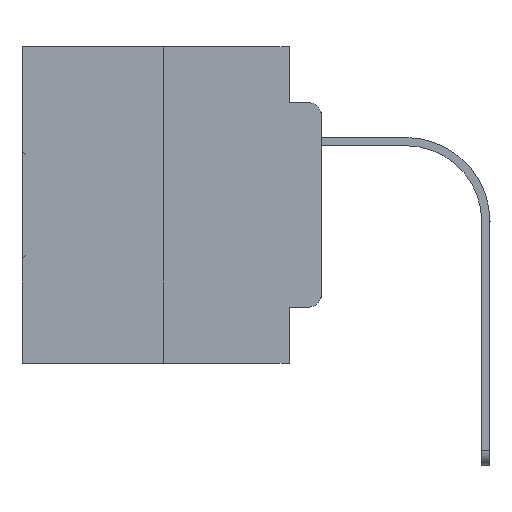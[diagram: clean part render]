
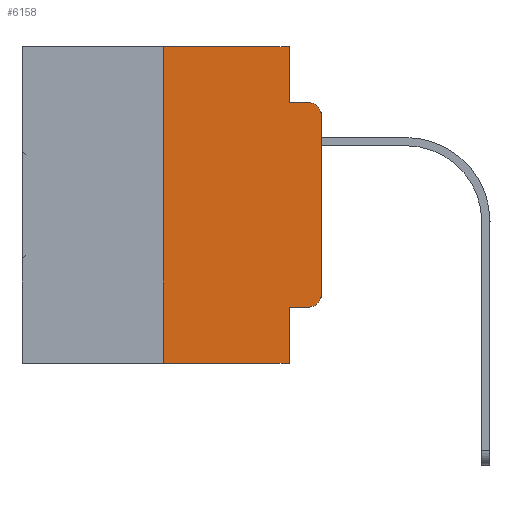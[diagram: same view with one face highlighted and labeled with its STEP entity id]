
A CAD part, left-side view. The second image highlights one B-rep face of the part: STEP entity #6158.
In plain terms, the highlighted planar face has unit normal (-1, 0, 0).
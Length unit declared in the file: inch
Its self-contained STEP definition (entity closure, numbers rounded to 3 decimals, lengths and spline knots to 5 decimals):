
#133 = EDGE_CURVE ( 'NONE', #17402, #2380, #21622, .T. ) ;
#395 = VECTOR ( 'NONE', #9404, 39.37008 ) ;
#664 = CARTESIAN_POINT ( 'NONE',  ( 0., 0.25, 0. ) ) ;
#854 = LINE ( 'NONE', #12624, #10473 ) ;
#1053 = EDGE_CURVE ( 'NONE', #10923, #3500, #10325, .T. ) ;
#1316 = DIRECTION ( 'NONE',  ( 0., 0., 1. ) ) ;
#1574 = VECTOR ( 'NONE', #30043, 39.37008 ) ;
#2047 = ORIENTED_EDGE ( 'NONE', *, *, #26265, .T. ) ;
#2172 = CARTESIAN_POINT ( 'NONE',  ( 0., 0., -0.1085 ) ) ;
#2380 = VERTEX_POINT ( 'NONE', #4368 ) ;
#2775 = EDGE_CURVE ( 'NONE', #23478, #12491, #9440, .T. ) ;
#3223 = EDGE_CURVE ( 'NONE', #12491, #11195, #23045, .T. ) ;
#3500 = VERTEX_POINT ( 'NONE', #2172 ) ;
#3657 = EDGE_CURVE ( 'NONE', #11195, #26979, #28485, .T. ) ;
#4109 = LINE ( 'NONE', #8973, #10966 ) ;
#4368 = CARTESIAN_POINT ( 'NONE',  ( 0., 0.051, -0.5 ) ) ;
#6158 = ADVANCED_FACE ( 'NONE', ( #27324 ), #6329, .F. ) ;
#6208 = ORIENTED_EDGE ( 'NONE', *, *, #1053, .T. ) ;
#6329 = PLANE ( 'NONE',  #11194 ) ;
#6498 = DIRECTION ( 'NONE',  ( -1., 0., 0. ) ) ;
#7035 = ORIENTED_EDGE ( 'NONE', *, *, #133, .F. ) ;
#7985 = LINE ( 'NONE', #17350, #1574 ) ;
#8927 = CARTESIAN_POINT ( 'NONE',  ( 0., 0.473, 0. ) ) ;
#8973 = CARTESIAN_POINT ( 'NONE',  ( 0., 0.25, 0. ) ) ;
#9230 = DIRECTION ( 'NONE',  ( -1., 0., 0. ) ) ;
#9243 = CARTESIAN_POINT ( 'NONE',  ( 0., 0.051, 0. ) ) ;
#9404 = DIRECTION ( 'NONE',  ( 0., 0., -1. ) ) ;
#9440 = LINE ( 'NONE', #26138, #26828 ) ;
#9497 = CIRCLE ( 'NONE', #17349, 0.02 ) ;
#9725 = CARTESIAN_POINT ( 'NONE',  ( 0., 0.051, 0. ) ) ;
#10325 = LINE ( 'NONE', #24876, #26907 ) ;
#10331 = CIRCLE ( 'NONE', #17681, 0.02 ) ;
#10473 = VECTOR ( 'NONE', #21947, 39.37008 ) ;
#10923 = VERTEX_POINT ( 'NONE', #30077 ) ;
#10943 = EDGE_CURVE ( 'NONE', #3500, #26979, #10331, .T. ) ;
#10966 = VECTOR ( 'NONE', #13126, 39.37008 ) ;
#11194 = AXIS2_PLACEMENT_3D ( 'NONE', #8927, #15665, #25036 ) ;
#11195 = VERTEX_POINT ( 'NONE', #17194 ) ;
#11224 = EDGE_CURVE ( 'NONE', #28524, #2380, #7985, .T. ) ;
#11507 = ORIENTED_EDGE ( 'NONE', *, *, #3223, .F. ) ;
#11794 = ORIENTED_EDGE ( 'NONE', *, *, #11224, .T. ) ;
#12491 = VERTEX_POINT ( 'NONE', #9725 ) ;
#12624 = CARTESIAN_POINT ( 'NONE',  ( 0., 0.051, -0.4115 ) ) ;
#13034 = CARTESIAN_POINT ( 'NONE',  ( 0., 0.051, -0.4115 ) ) ;
#13126 = DIRECTION ( 'NONE',  ( 0., 0., 1. ) ) ;
#13244 = CARTESIAN_POINT ( 'NONE',  ( 0., 0.02, -0.3915 ) ) ;
#13622 = CARTESIAN_POINT ( 'NONE',  ( 0., 0.25, -0.5 ) ) ;
#15005 = ORIENTED_EDGE ( 'NONE', *, *, #10943, .T. ) ;
#15176 = CARTESIAN_POINT ( 'NONE',  ( 0., 0.051, 0. ) ) ;
#15540 = EDGE_CURVE ( 'NONE', #28363, #10923, #9497, .T. ) ;
#15665 = DIRECTION ( 'NONE',  ( 1., 0., 0. ) ) ;
#16259 = VECTOR ( 'NONE', #26185, 39.37008 ) ;
#17194 = CARTESIAN_POINT ( 'NONE',  ( 0., 0.051, -0.0885 ) ) ;
#17349 = AXIS2_PLACEMENT_3D ( 'NONE', #13244, #6498, #29330 ) ;
#17350 = CARTESIAN_POINT ( 'NONE',  ( 0., 0.473, -0.5 ) ) ;
#17402 = VERTEX_POINT ( 'NONE', #13034 ) ;
#17681 = AXIS2_PLACEMENT_3D ( 'NONE', #21025, #9230, #25787 ) ;
#17783 = ORIENTED_EDGE ( 'NONE', *, *, #15540, .T. ) ;
#17992 = ORIENTED_EDGE ( 'NONE', *, *, #2775, .F. ) ;
#18763 = DIRECTION ( 'NONE',  ( 0., -1., 0. ) ) ;
#19274 = CARTESIAN_POINT ( 'NONE',  ( 0., 0.02, -0.0885 ) ) ;
#20689 = EDGE_LOOP ( 'NONE', ( #6208, #15005, #23665, #11507, #17992, #25135, #11794, #7035, #2047, #17783 ) ) ;
#21025 = CARTESIAN_POINT ( 'NONE',  ( 0., 0.02, -0.1085 ) ) ;
#21277 = CARTESIAN_POINT ( 'NONE',  ( 0., 0.051, -0.0885 ) ) ;
#21622 = LINE ( 'NONE', #15176, #22455 ) ;
#21947 = DIRECTION ( 'NONE',  ( 0., -1., 0. ) ) ;
#22455 = VECTOR ( 'NONE', #28682, 39.37008 ) ;
#23045 = LINE ( 'NONE', #9243, #395 ) ;
#23478 = VERTEX_POINT ( 'NONE', #664 ) ;
#23665 = ORIENTED_EDGE ( 'NONE', *, *, #3657, .F. ) ;
#24876 = CARTESIAN_POINT ( 'NONE',  ( 0., 0., 0. ) ) ;
#25036 = DIRECTION ( 'NONE',  ( 0., 0., -1. ) ) ;
#25135 = ORIENTED_EDGE ( 'NONE', *, *, #25958, .F. ) ;
#25787 = DIRECTION ( 'NONE',  ( 0., 0., -1. ) ) ;
#25958 = EDGE_CURVE ( 'NONE', #28524, #23478, #4109, .T. ) ;
#26138 = CARTESIAN_POINT ( 'NONE',  ( 0., 0.473, 0. ) ) ;
#26185 = DIRECTION ( 'NONE',  ( 0., -1., 0. ) ) ;
#26265 = EDGE_CURVE ( 'NONE', #17402, #28363, #854, .T. ) ;
#26828 = VECTOR ( 'NONE', #18763, 39.37008 ) ;
#26907 = VECTOR ( 'NONE', #1316, 39.37008 ) ;
#26979 = VERTEX_POINT ( 'NONE', #19274 ) ;
#27324 = FACE_OUTER_BOUND ( 'NONE', #20689, .T. ) ;
#28363 = VERTEX_POINT ( 'NONE', #29572 ) ;
#28485 = LINE ( 'NONE', #21277, #16259 ) ;
#28524 = VERTEX_POINT ( 'NONE', #13622 ) ;
#28682 = DIRECTION ( 'NONE',  ( 0., 0., -1. ) ) ;
#29330 = DIRECTION ( 'NONE',  ( 0., 0., -1. ) ) ;
#29572 = CARTESIAN_POINT ( 'NONE',  ( 0., 0.02, -0.4115 ) ) ;
#30043 = DIRECTION ( 'NONE',  ( 0., -1., 0. ) ) ;
#30077 = CARTESIAN_POINT ( 'NONE',  ( 0., 0., -0.3915 ) ) ;
